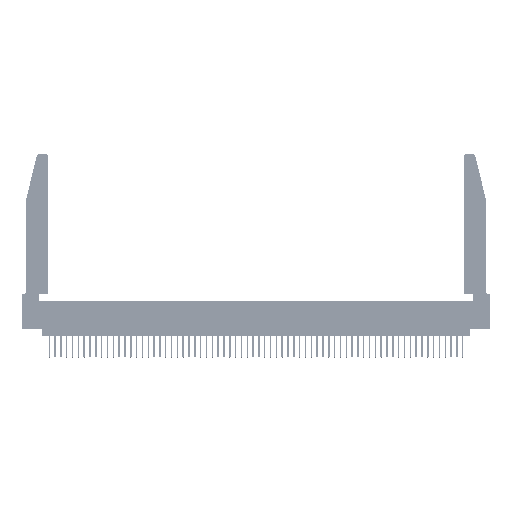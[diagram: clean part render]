
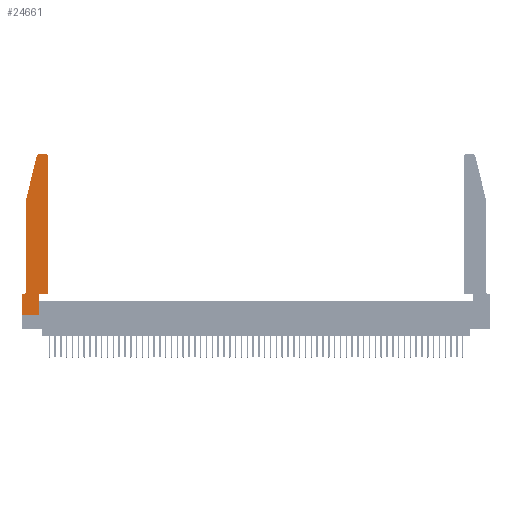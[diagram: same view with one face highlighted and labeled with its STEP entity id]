
A CAD part, top view. The second image highlights one B-rep face of the part: STEP entity #24661.
In plain terms, the highlighted planar face has unit normal (0, 0, 1).
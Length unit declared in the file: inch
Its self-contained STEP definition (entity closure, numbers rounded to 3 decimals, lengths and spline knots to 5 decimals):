
#358 = EDGE_CURVE ( 'NONE', #23652, #12527, #48790, .T. ) ;
#2661 = LINE ( 'NONE', #38027, #36870 ) ;
#3083 = VERTEX_POINT ( 'NONE', #13130 ) ;
#3886 = PLANE ( 'NONE',  #26831 ) ;
#6430 = VERTEX_POINT ( 'NONE', #12670 ) ;
#6576 = CARTESIAN_POINT ( 'NONE',  ( 0.0755, 2., 0.37 ) ) ;
#6747 = CARTESIAN_POINT ( 'NONE',  ( 0.0055, 0.42, 0.37 ) ) ;
#7807 = EDGE_CURVE ( 'NONE', #9080, #23652, #43193, .T. ) ;
#8404 = DIRECTION ( 'NONE',  ( 1., 0., 0. ) ) ;
#9080 = VERTEX_POINT ( 'NONE', #16316 ) ;
#9087 = CARTESIAN_POINT ( 'NONE',  ( 0.25487, 2.72718, 0.37 ) ) ;
#9247 = VECTOR ( 'NONE', #56791, 39.37008 ) ;
#9619 = EDGE_CURVE ( 'NONE', #14920, #24745, #2661, .T. ) ;
#9862 = ORIENTED_EDGE ( 'NONE', *, *, #9619, .T. ) ;
#10726 = LINE ( 'NONE', #11082, #34432 ) ;
#11009 = DIRECTION ( 'NONE',  ( 0., 0., 1. ) ) ;
#11082 = CARTESIAN_POINT ( 'NONE',  ( 0.0755, 2., 0.37 ) ) ;
#11258 = DIRECTION ( 'NONE',  ( -1., 0., 0. ) ) ;
#11433 = VECTOR ( 'NONE', #33013, 39.37008 ) ;
#12527 = VERTEX_POINT ( 'NONE', #35763 ) ;
#12670 = CARTESIAN_POINT ( 'NONE',  ( 0.4205, 2.75, 0.37 ) ) ;
#13130 = CARTESIAN_POINT ( 'NONE',  ( 0.284, 2.75, 0.37 ) ) ;
#13417 = ORIENTED_EDGE ( 'NONE', *, *, #48126, .T. ) ;
#14333 = LINE ( 'NONE', #44037, #22001 ) ;
#14920 = VERTEX_POINT ( 'NONE', #53721 ) ;
#15379 = ORIENTED_EDGE ( 'NONE', *, *, #35041, .T. ) ;
#15611 = DIRECTION ( 'NONE',  ( -1., 0., 0. ) ) ;
#15864 = DIRECTION ( 'NONE',  ( 0., 1., 0. ) ) ;
#16316 = CARTESIAN_POINT ( 'NONE',  ( 0.0055, 0.35, 0.37 ) ) ;
#16933 = CARTESIAN_POINT ( 'NONE',  ( 0.4505, 2.72, 0.37 ) ) ;
#17013 = EDGE_CURVE ( 'NONE', #42466, #6430, #50211, .T. ) ;
#17245 = ORIENTED_EDGE ( 'NONE', *, *, #52480, .T. ) ;
#17782 = LINE ( 'NONE', #42165, #41331 ) ;
#18272 = VECTOR ( 'NONE', #51582, 39.37008 ) ;
#21086 = CARTESIAN_POINT ( 'NONE',  ( 0.284, 2.72, 0.37 ) ) ;
#21588 = CARTESIAN_POINT ( 'NONE',  ( 0.4505, 0.35, 0.37 ) ) ;
#22001 = VECTOR ( 'NONE', #48627, 39.37008 ) ;
#22550 = LINE ( 'NONE', #21588, #9247 ) ;
#22723 = FACE_OUTER_BOUND ( 'NONE', #54420, .T. ) ;
#23652 = VERTEX_POINT ( 'NONE', #28803 ) ;
#24411 = CARTESIAN_POINT ( 'NONE',  ( 0.4505, 0.35, 0.37 ) ) ;
#24661 = ADVANCED_FACE ( 'NONE', ( #22723 ), #3886, .T. ) ;
#24711 = LINE ( 'NONE', #50670, #11433 ) ;
#24745 = VERTEX_POINT ( 'NONE', #40077 ) ;
#25225 = CARTESIAN_POINT ( 'NONE',  ( 0.0755, 0.35, 0.37 ) ) ;
#25482 = ORIENTED_EDGE ( 'NONE', *, *, #26002, .T. ) ;
#25557 = EDGE_CURVE ( 'NONE', #28532, #45885, #10726, .T. ) ;
#25562 = DIRECTION ( 'NONE',  ( 1., 0., 0. ) ) ;
#26002 = EDGE_CURVE ( 'NONE', #39174, #42466, #22550, .T. ) ;
#26086 = ORIENTED_EDGE ( 'NONE', *, *, #25557, .T. ) ;
#26831 = AXIS2_PLACEMENT_3D ( 'NONE', #30662, #35109, #8404 ) ;
#27120 = ORIENTED_EDGE ( 'NONE', *, *, #358, .T. ) ;
#27139 = EDGE_CURVE ( 'NONE', #3083, #29914, #32973, .T. ) ;
#28532 = VERTEX_POINT ( 'NONE', #52352 ) ;
#28803 = CARTESIAN_POINT ( 'NONE',  ( 0., 0.35, 0.37 ) ) ;
#29914 = VERTEX_POINT ( 'NONE', #9087 ) ;
#30662 = CARTESIAN_POINT ( 'NONE',  ( 0., 0.35, 0.37 ) ) ;
#31007 = AXIS2_PLACEMENT_3D ( 'NONE', #21086, #51935, #25562 ) ;
#31761 = ORIENTED_EDGE ( 'NONE', *, *, #33292, .T. ) ;
#32973 = CIRCLE ( 'NONE', #31007, 0.03 ) ;
#33013 = DIRECTION ( 'NONE',  ( 1., 0., 0. ) ) ;
#33284 = DIRECTION ( 'NONE',  ( -0.239, -0.971, 0. ) ) ;
#33292 = EDGE_CURVE ( 'NONE', #12527, #14920, #24711, .T. ) ;
#34432 = VECTOR ( 'NONE', #42135, 39.37008 ) ;
#34778 = CIRCLE ( 'NONE', #43426, 0.07 ) ;
#35041 = EDGE_CURVE ( 'NONE', #29914, #28532, #36690, .T. ) ;
#35109 = DIRECTION ( 'NONE',  ( 0., 0., 1. ) ) ;
#35763 = CARTESIAN_POINT ( 'NONE',  ( 0., 0., 0.37 ) ) ;
#36690 = LINE ( 'NONE', #6576, #57189 ) ;
#36870 = VECTOR ( 'NONE', #15864, 39.37008 ) ;
#37170 = VECTOR ( 'NONE', #51324, 39.37008 ) ;
#37674 = CARTESIAN_POINT ( 'NONE',  ( 0.4205, 2.72, 0.37 ) ) ;
#37921 = DIRECTION ( 'NONE',  ( 0., 0., -1. ) ) ;
#38027 = CARTESIAN_POINT ( 'NONE',  ( 0.2865, 0.35, 0.37 ) ) ;
#38132 = CARTESIAN_POINT ( 'NONE',  ( 0., 0., 0.37 ) ) ;
#38999 = ORIENTED_EDGE ( 'NONE', *, *, #56052, .T. ) ;
#39174 = VERTEX_POINT ( 'NONE', #24411 ) ;
#40077 = CARTESIAN_POINT ( 'NONE',  ( 0.2865, 0.35, 0.37 ) ) ;
#41193 = CARTESIAN_POINT ( 'NONE',  ( 0.0755, 0.42, 0.37 ) ) ;
#41331 = VECTOR ( 'NONE', #15611, 39.37008 ) ;
#42066 = DIRECTION ( 'NONE',  ( 1., 0., 0. ) ) ;
#42135 = DIRECTION ( 'NONE',  ( 0., -1., 0. ) ) ;
#42165 = CARTESIAN_POINT ( 'NONE',  ( 0.2605, 2.75, 0.37 ) ) ;
#42466 = VERTEX_POINT ( 'NONE', #16933 ) ;
#43193 = LINE ( 'NONE', #25225, #18272 ) ;
#43426 = AXIS2_PLACEMENT_3D ( 'NONE', #6747, #37921, #11258 ) ;
#44037 = CARTESIAN_POINT ( 'NONE',  ( 0.4505, 0.35, 0.37 ) ) ;
#45885 = VERTEX_POINT ( 'NONE', #41193 ) ;
#48126 = EDGE_CURVE ( 'NONE', #6430, #3083, #17782, .T. ) ;
#48187 = ORIENTED_EDGE ( 'NONE', *, *, #17013, .T. ) ;
#48627 = DIRECTION ( 'NONE',  ( 1., 0., 0. ) ) ;
#48790 = LINE ( 'NONE', #38132, #37170 ) ;
#50211 = CIRCLE ( 'NONE', #54962, 0.03 ) ;
#50232 = ORIENTED_EDGE ( 'NONE', *, *, #7807, .T. ) ;
#50670 = CARTESIAN_POINT ( 'NONE',  ( 0., 0., 0.37 ) ) ;
#51324 = DIRECTION ( 'NONE',  ( 0., -1., 0. ) ) ;
#51582 = DIRECTION ( 'NONE',  ( -1., 0., 0. ) ) ;
#51935 = DIRECTION ( 'NONE',  ( 0., 0., 1. ) ) ;
#52352 = CARTESIAN_POINT ( 'NONE',  ( 0.0755, 2., 0.37 ) ) ;
#52480 = EDGE_CURVE ( 'NONE', #24745, #39174, #14333, .T. ) ;
#52804 = ORIENTED_EDGE ( 'NONE', *, *, #27139, .T. ) ;
#53721 = CARTESIAN_POINT ( 'NONE',  ( 0.2865, 0., 0.37 ) ) ;
#54420 = EDGE_LOOP ( 'NONE', ( #13417, #52804, #15379, #26086, #38999, #50232, #27120, #31761, #9862, #17245, #25482, #48187 ) ) ;
#54962 = AXIS2_PLACEMENT_3D ( 'NONE', #37674, #11009, #42066 ) ;
#56052 = EDGE_CURVE ( 'NONE', #45885, #9080, #34778, .T. ) ;
#56791 = DIRECTION ( 'NONE',  ( 0., 1., 0. ) ) ;
#57189 = VECTOR ( 'NONE', #33284, 39.37008 ) ;
